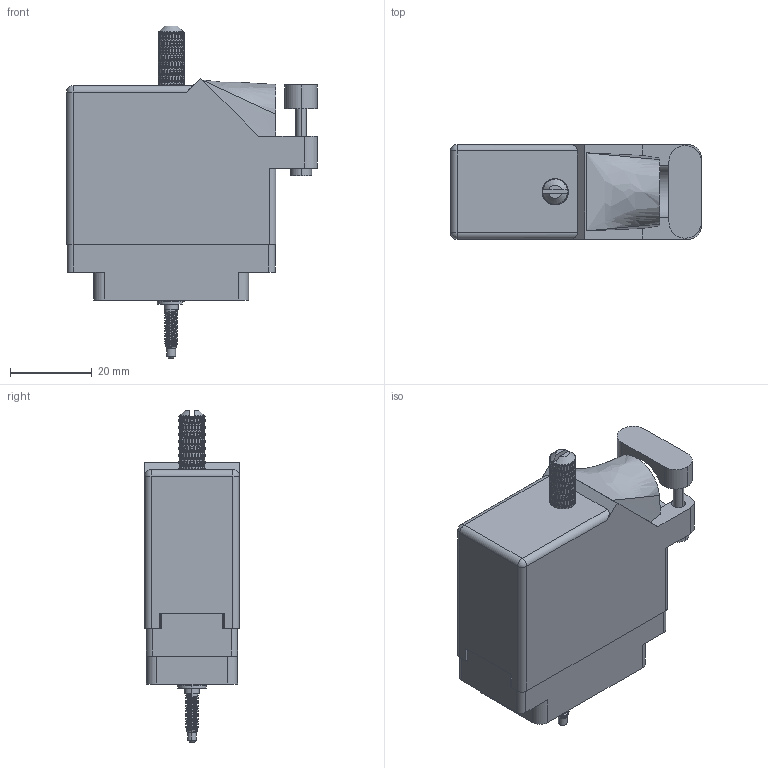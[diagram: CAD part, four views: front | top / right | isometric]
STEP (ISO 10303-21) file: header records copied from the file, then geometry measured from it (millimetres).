
FILE_DESCRIPTION (( 'STEP AP203' ), '1' );
FILE_NAME ('519-036-500-325.STEP', '2020-03-02T21:53:36', ( '' ), ( '' ), 'SwSTEP 2.0', 'SolidWorks 2016', '' );
FILE_SCHEMA (( 'CONFIG_CONTROL_DESIGN' ));
Products named in the file (9): 519-036-500-325; 516-230-001_Plastic - 038 Side Entry; 516-251-035-100; Actuating Screw Assy 038-056; 516-253-035-100; 516-292-001_500 Contact; 519 Plug Insulator_036; 516-250-038-111; 516-253-138-107
Assembly tree (44 placements, depth 3):
  519-036-500-325
    519 Plug Insulator_036
    516-292-001_500 Contact  x36
    Actuating Screw Assy 038-056
      516-251-035-100
      516-253-035-100  x2
      516-253-138-107
      516-250-038-111
    516-230-001_Plastic - 038 Side Entry
Bounding box: 61.21 x 23.11 x 81.03 mm (x, y, z)
Volume: 22899.6 mm3; surface area: 33975.5 mm2
Topology: 43 solids, 43 shells, 5062 faces, 13615 edges, 8662 vertices
Faces by surface type: plane 2276, cylinder 1539, bspline 1225, cone 20, sphere 2
Entity records: 101841 total; most frequent: CARTESIAN_POINT 54430, ORIENTED_EDGE 11802, DIRECTION 6969, EDGE_CURVE 5901, VERTEX_POINT 3544, EDGE_LOOP 2521, ADVANCED_FACE 2396, FACE_OUTER_BOUND 2396
